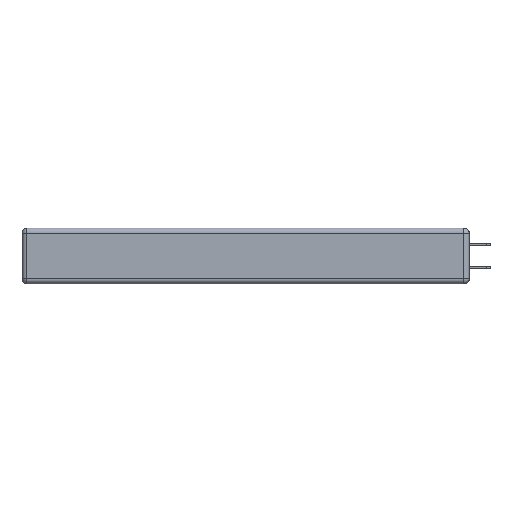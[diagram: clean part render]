
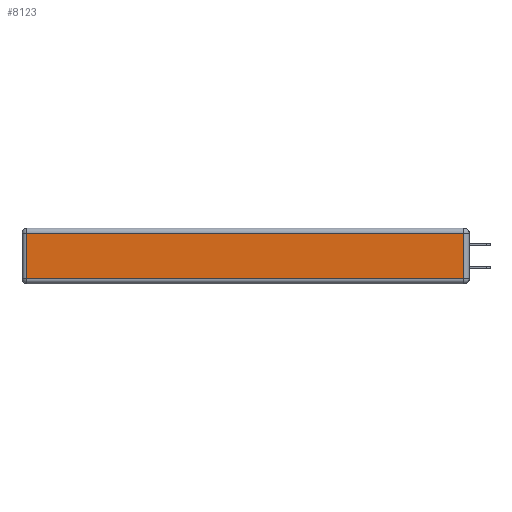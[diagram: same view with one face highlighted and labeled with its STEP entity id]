
A CAD part, left-side view. The second image highlights one B-rep face of the part: STEP entity #8123.
In plain terms, the highlighted planar face has unit normal (-1, 0, 0).
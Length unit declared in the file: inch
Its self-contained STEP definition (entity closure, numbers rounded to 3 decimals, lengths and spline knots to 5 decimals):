
#139 = PLANE ( 'NONE',  #2592 ) ;
#1507 = LINE ( 'NONE', #2648, #16812 ) ;
#1709 = FACE_OUTER_BOUND ( 'NONE', #8796, .T. ) ;
#2592 = AXIS2_PLACEMENT_3D ( 'NONE', #16040, #2994, #12544 ) ;
#2648 = CARTESIAN_POINT ( 'NONE',  ( 0., 0., -0.313 ) ) ;
#2885 = DIRECTION ( 'NONE',  ( 0., 0., -1. ) ) ;
#2975 = CARTESIAN_POINT ( 'NONE',  ( 0., 0.03, -0.03 ) ) ;
#2994 = DIRECTION ( 'NONE',  ( -1., 0., 0. ) ) ;
#3370 = LINE ( 'NONE', #4121, #10720 ) ;
#4121 = CARTESIAN_POINT ( 'NONE',  ( 0., 2.72, -0.343 ) ) ;
#4582 = ORIENTED_EDGE ( 'NONE', *, *, #7964, .T. ) ;
#5027 = VECTOR ( 'NONE', #9980, 39.37008 ) ;
#5623 = CARTESIAN_POINT ( 'NONE',  ( 0., 2.72, -0.313 ) ) ;
#5641 = LINE ( 'NONE', #11559, #10640 ) ;
#6178 = CARTESIAN_POINT ( 'NONE',  ( 0., 0.03, -0.313 ) ) ;
#6564 = VERTEX_POINT ( 'NONE', #16824 ) ;
#7575 = VERTEX_POINT ( 'NONE', #5623 ) ;
#7964 = EDGE_CURVE ( 'NONE', #6564, #7575, #3370, .T. ) ;
#8123 = ADVANCED_FACE ( 'NONE', ( #1709 ), #139, .T. ) ;
#8796 = EDGE_LOOP ( 'NONE', ( #15293, #12029, #10595, #4582 ) ) ;
#8831 = CARTESIAN_POINT ( 'NONE',  ( 0., 2.75, -0.03 ) ) ;
#9325 = EDGE_CURVE ( 'NONE', #17081, #6564, #15101, .T. ) ;
#9980 = DIRECTION ( 'NONE',  ( 0., 1., 0. ) ) ;
#10595 = ORIENTED_EDGE ( 'NONE', *, *, #9325, .T. ) ;
#10640 = VECTOR ( 'NONE', #11430, 39.37008 ) ;
#10720 = VECTOR ( 'NONE', #2885, 39.37008 ) ;
#10867 = VERTEX_POINT ( 'NONE', #6178 ) ;
#11430 = DIRECTION ( 'NONE',  ( 0., 0., 1. ) ) ;
#11559 = CARTESIAN_POINT ( 'NONE',  ( 0., 0.03, -0.343 ) ) ;
#11607 = EDGE_CURVE ( 'NONE', #7575, #10867, #1507, .T. ) ;
#12029 = ORIENTED_EDGE ( 'NONE', *, *, #14243, .T. ) ;
#12205 = DIRECTION ( 'NONE',  ( 0., -1., 0. ) ) ;
#12544 = DIRECTION ( 'NONE',  ( 0., 0., 1. ) ) ;
#14243 = EDGE_CURVE ( 'NONE', #10867, #17081, #5641, .T. ) ;
#15101 = LINE ( 'NONE', #8831, #5027 ) ;
#15293 = ORIENTED_EDGE ( 'NONE', *, *, #11607, .T. ) ;
#16040 = CARTESIAN_POINT ( 'NONE',  ( 0., 0., -0.343 ) ) ;
#16812 = VECTOR ( 'NONE', #12205, 39.37008 ) ;
#16824 = CARTESIAN_POINT ( 'NONE',  ( 0., 2.72, -0.03 ) ) ;
#17081 = VERTEX_POINT ( 'NONE', #2975 ) ;
